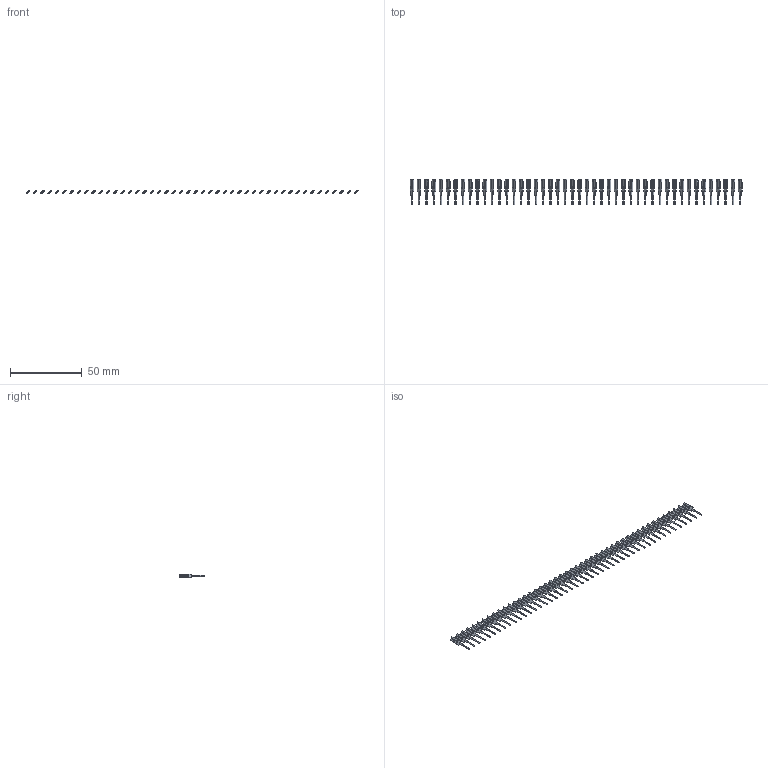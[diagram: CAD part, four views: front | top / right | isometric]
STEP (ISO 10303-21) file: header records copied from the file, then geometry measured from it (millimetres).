
FILE_DESCRIPTION (( 'STEP AP203' ), '1' );
FILE_NAME ('106-046-251-200.STEP', '2020-04-16T20:24:43', ( '' ), ( '' ), 'SwSTEP 2.0', 'SolidWorks 2016', '' );
FILE_SCHEMA (( 'CONFIG_CONTROL_DESIGN' ));
Length unit declared in the file: inch
Products named in the file (2): 106-046-251-200; 100-290-001_100-290-251
Assembly tree (46 placements, depth 2):
  106-046-251-200
    100-290-001_100-290-251  x46
Bounding box: 231.13 x 17.9 x 2.53 mm (x, y, z)
Volume: 841 mm3; surface area: 4133.9 mm2
Topology: 46 solids, 46 shells, 1288 faces, 3588 edges, 2392 vertices
Faces by surface type: plane 1012, cylinder 276
Entity records: 2534 total; most frequent: DIRECTION 240, CARTESIAN_POINT 219, ORIENTED_EDGE 156, CALENDAR_DATE 102, COORDINATED_UNIVERSAL_TIME_OFFSET 102, DATE_AND_TIME 102, LOCAL_TIME 102, AXIS2_PLACEMENT_3D 89
